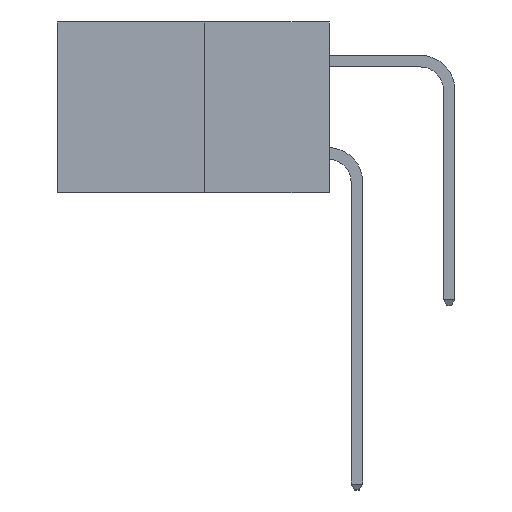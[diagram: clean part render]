
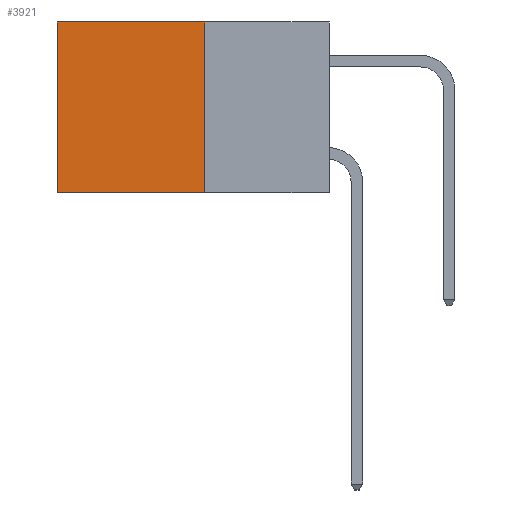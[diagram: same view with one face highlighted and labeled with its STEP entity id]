
A CAD part, left-side view. The second image highlights one B-rep face of the part: STEP entity #3921.
In plain terms, the highlighted planar face has unit normal (-1, 0, 0).
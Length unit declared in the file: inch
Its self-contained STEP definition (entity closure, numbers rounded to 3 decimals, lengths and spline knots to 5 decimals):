
#236 = VECTOR ( 'NONE', #426, 39.37008 ) ;
#426 = DIRECTION ( 'NONE',  ( 0., 1., 0. ) ) ;
#1063 = CARTESIAN_POINT ( 'NONE',  ( 0.277, 0.59, -0.37 ) ) ;
#1240 = VERTEX_POINT ( 'NONE', #1063 ) ;
#1524 = CARTESIAN_POINT ( 'NONE',  ( 0.277, 0.27, 0. ) ) ;
#1648 = ORIENTED_EDGE ( 'NONE', *, *, #8903, .T. ) ;
#1843 = AXIS2_PLACEMENT_3D ( 'NONE', #8527, #8809, #8299 ) ;
#2322 = ORIENTED_EDGE ( 'NONE', *, *, #4995, .F. ) ;
#2609 = FACE_OUTER_BOUND ( 'NONE', #3793, .T. ) ;
#2751 = VERTEX_POINT ( 'NONE', #1524 ) ;
#2836 = ORIENTED_EDGE ( 'NONE', *, *, #9508, .F. ) ;
#3140 = VERTEX_POINT ( 'NONE', #6355 ) ;
#3149 = CARTESIAN_POINT ( 'NONE',  ( 0.277, 0.27, 0. ) ) ;
#3180 = ORIENTED_EDGE ( 'NONE', *, *, #7347, .T. ) ;
#3310 = VECTOR ( 'NONE', #10125, 39.37008 ) ;
#3565 = LINE ( 'NONE', #3149, #3310 ) ;
#3687 = VERTEX_POINT ( 'NONE', #9540 ) ;
#3793 = EDGE_LOOP ( 'NONE', ( #3180, #2836, #2322, #1648 ) ) ;
#3921 = ADVANCED_FACE ( 'NONE', ( #2609 ), #8469, .F. ) ;
#4165 = VECTOR ( 'NONE', #6453, 39.37008 ) ;
#4995 = EDGE_CURVE ( 'NONE', #2751, #3687, #10038, .T. ) ;
#6201 = CARTESIAN_POINT ( 'NONE',  ( 0.277, 0.27, -0.37 ) ) ;
#6314 = VECTOR ( 'NONE', #8610, 39.37008 ) ;
#6340 = CARTESIAN_POINT ( 'NONE',  ( 0.277, 0.59, -0.37 ) ) ;
#6355 = CARTESIAN_POINT ( 'NONE',  ( 0.277, 0.59, 0. ) ) ;
#6453 = DIRECTION ( 'NONE',  ( 0., 0., -1. ) ) ;
#6903 = LINE ( 'NONE', #9979, #236 ) ;
#7347 = EDGE_CURVE ( 'NONE', #3140, #1240, #8555, .T. ) ;
#8299 = DIRECTION ( 'NONE',  ( 0., 0., -1. ) ) ;
#8469 = PLANE ( 'NONE',  #1843 ) ;
#8527 = CARTESIAN_POINT ( 'NONE',  ( 0.277, 0.27, -0.37 ) ) ;
#8555 = LINE ( 'NONE', #6340, #6314 ) ;
#8610 = DIRECTION ( 'NONE',  ( 0., 0., -1. ) ) ;
#8809 = DIRECTION ( 'NONE',  ( 1., 0., 0. ) ) ;
#8903 = EDGE_CURVE ( 'NONE', #2751, #3140, #3565, .T. ) ;
#9508 = EDGE_CURVE ( 'NONE', #3687, #1240, #6903, .T. ) ;
#9540 = CARTESIAN_POINT ( 'NONE',  ( 0.277, 0.27, -0.37 ) ) ;
#9979 = CARTESIAN_POINT ( 'NONE',  ( 0.277, 0.27, -0.37 ) ) ;
#10038 = LINE ( 'NONE', #6201, #4165 ) ;
#10125 = DIRECTION ( 'NONE',  ( 0., 1., 0. ) ) ;
